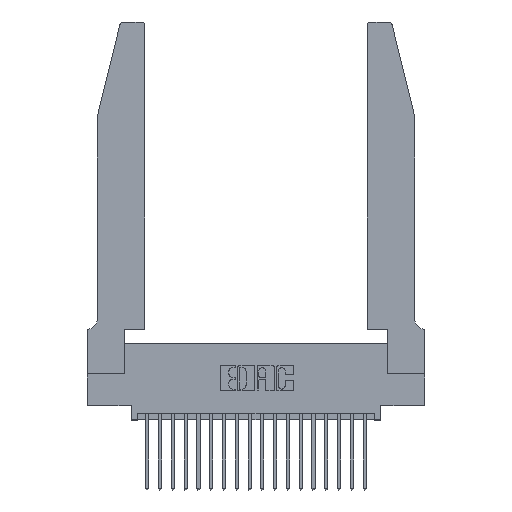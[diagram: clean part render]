
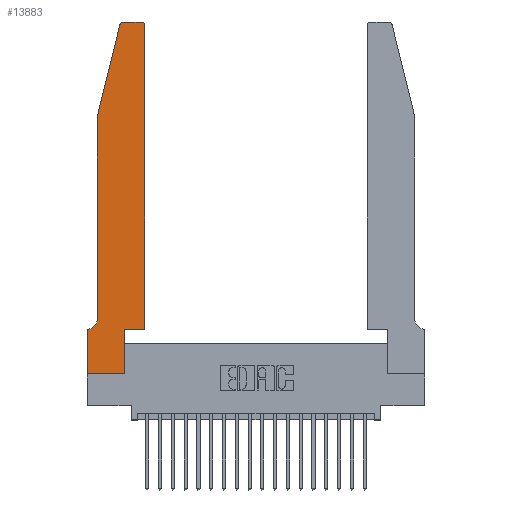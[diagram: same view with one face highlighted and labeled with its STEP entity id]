
A CAD part, top view. The second image highlights one B-rep face of the part: STEP entity #13883.
In plain terms, the highlighted planar face has unit normal (0, 0, 1).
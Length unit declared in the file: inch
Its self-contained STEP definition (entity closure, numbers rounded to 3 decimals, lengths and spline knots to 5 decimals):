
#128 = CARTESIAN_POINT ( 'NONE',  ( 0., 0.35, 0.37 ) ) ;
#136 = EDGE_CURVE ( 'NONE', #1416, #998, #16608, .T. ) ;
#261 = AXIS2_PLACEMENT_3D ( 'NONE', #13295, #6461, #11651 ) ;
#364 = VECTOR ( 'NONE', #13575, 39.37008 ) ;
#492 = VECTOR ( 'NONE', #21256, 39.37008 ) ;
#529 = DIRECTION ( 'NONE',  ( 1., 0., 0. ) ) ;
#576 = ORIENTED_EDGE ( 'NONE', *, *, #10996, .T. ) ;
#998 = VERTEX_POINT ( 'NONE', #2997 ) ;
#1009 = CARTESIAN_POINT ( 'NONE',  ( 0.284, 2.75, 0.37 ) ) ;
#1416 = VERTEX_POINT ( 'NONE', #128 ) ;
#1427 = DIRECTION ( 'NONE',  ( 0., 0., -1. ) ) ;
#1960 = CARTESIAN_POINT ( 'NONE',  ( 0.4505, 2.72, 0.37 ) ) ;
#2762 = EDGE_CURVE ( 'NONE', #20988, #3306, #14100, .T. ) ;
#2997 = CARTESIAN_POINT ( 'NONE',  ( 0., 0., 0.37 ) ) ;
#3073 = DIRECTION ( 'NONE',  ( -1., 0., 0. ) ) ;
#3126 = CARTESIAN_POINT ( 'NONE',  ( 0.0755, 0.35, 0.37 ) ) ;
#3306 = VERTEX_POINT ( 'NONE', #5013 ) ;
#3954 = CARTESIAN_POINT ( 'NONE',  ( 0.25487, 2.72718, 0.37 ) ) ;
#4302 = ORIENTED_EDGE ( 'NONE', *, *, #16537, .T. ) ;
#4662 = VERTEX_POINT ( 'NONE', #20462 ) ;
#4788 = VERTEX_POINT ( 'NONE', #1009 ) ;
#5013 = CARTESIAN_POINT ( 'NONE',  ( 0.2865, 0.35, 0.37 ) ) ;
#5222 = ORIENTED_EDGE ( 'NONE', *, *, #2762, .T. ) ;
#5242 = DIRECTION ( 'NONE',  ( -1., 0., 0. ) ) ;
#5461 = CARTESIAN_POINT ( 'NONE',  ( 0.2865, 0., 0.37 ) ) ;
#5582 = CARTESIAN_POINT ( 'NONE',  ( 0.4205, 2.75, 0.37 ) ) ;
#5585 = LINE ( 'NONE', #14156, #22278 ) ;
#5798 = ORIENTED_EDGE ( 'NONE', *, *, #12582, .T. ) ;
#5833 = CARTESIAN_POINT ( 'NONE',  ( 0.0755, 2., 0.37 ) ) ;
#6042 = DIRECTION ( 'NONE',  ( 1., 0., 0. ) ) ;
#6139 = AXIS2_PLACEMENT_3D ( 'NONE', #9614, #9840, #6042 ) ;
#6378 = EDGE_CURVE ( 'NONE', #6432, #14214, #9953, .T. ) ;
#6432 = VERTEX_POINT ( 'NONE', #11561 ) ;
#6461 = DIRECTION ( 'NONE',  ( 0., 0., 1. ) ) ;
#6501 = ORIENTED_EDGE ( 'NONE', *, *, #14180, .T. ) ;
#6626 = VECTOR ( 'NONE', #8017, 39.37008 ) ;
#7224 = CIRCLE ( 'NONE', #6139, 0.03 ) ;
#7790 = VECTOR ( 'NONE', #12864, 39.37008 ) ;
#8017 = DIRECTION ( 'NONE',  ( 0., 1., 0. ) ) ;
#8589 = FACE_OUTER_BOUND ( 'NONE', #19933, .T. ) ;
#8758 = CARTESIAN_POINT ( 'NONE',  ( 0.4505, 0.35, 0.37 ) ) ;
#9532 = VERTEX_POINT ( 'NONE', #1960 ) ;
#9598 = ORIENTED_EDGE ( 'NONE', *, *, #136, .T. ) ;
#9614 = CARTESIAN_POINT ( 'NONE',  ( 0.284, 2.72, 0.37 ) ) ;
#9824 = VERTEX_POINT ( 'NONE', #3954 ) ;
#9840 = DIRECTION ( 'NONE',  ( 0., 0., 1. ) ) ;
#9953 = CIRCLE ( 'NONE', #19726, 0.07 ) ;
#10314 = VECTOR ( 'NONE', #11611, 39.37008 ) ;
#10806 = VECTOR ( 'NONE', #14399, 39.37008 ) ;
#10824 = DIRECTION ( 'NONE',  ( -0.239, -0.971, 0. ) ) ;
#10859 = DIRECTION ( 'NONE',  ( 0., 0., 1. ) ) ;
#10996 = EDGE_CURVE ( 'NONE', #3306, #4662, #14779, .T. ) ;
#11364 = AXIS2_PLACEMENT_3D ( 'NONE', #21187, #10859, #529 ) ;
#11561 = CARTESIAN_POINT ( 'NONE',  ( 0.0755, 0.42, 0.37 ) ) ;
#11611 = DIRECTION ( 'NONE',  ( -1., 0., 0. ) ) ;
#11651 = DIRECTION ( 'NONE',  ( 1., 0., 0. ) ) ;
#12124 = ORIENTED_EDGE ( 'NONE', *, *, #14406, .T. ) ;
#12183 = LINE ( 'NONE', #20242, #364 ) ;
#12512 = DIRECTION ( 'NONE',  ( 0., -1., 0. ) ) ;
#12582 = EDGE_CURVE ( 'NONE', #4662, #9532, #18779, .T. ) ;
#12770 = VERTEX_POINT ( 'NONE', #13417 ) ;
#12864 = DIRECTION ( 'NONE',  ( 0., -1., 0. ) ) ;
#12946 = ORIENTED_EDGE ( 'NONE', *, *, #20002, .T. ) ;
#13025 = EDGE_CURVE ( 'NONE', #4788, #9824, #7224, .T. ) ;
#13295 = CARTESIAN_POINT ( 'NONE',  ( 0., 0.35, 0.37 ) ) ;
#13400 = CARTESIAN_POINT ( 'NONE',  ( 0.2865, 0.35, 0.37 ) ) ;
#13417 = CARTESIAN_POINT ( 'NONE',  ( 0.0755, 2., 0.37 ) ) ;
#13575 = DIRECTION ( 'NONE',  ( 1., 0., 0. ) ) ;
#13883 = ADVANCED_FACE ( 'NONE', ( #8589 ), #14917, .T. ) ;
#14091 = EDGE_CURVE ( 'NONE', #9532, #19957, #15506, .T. ) ;
#14100 = LINE ( 'NONE', #13400, #6626 ) ;
#14156 = CARTESIAN_POINT ( 'NONE',  ( 0.2605, 2.75, 0.37 ) ) ;
#14180 = EDGE_CURVE ( 'NONE', #19957, #4788, #5585, .T. ) ;
#14214 = VERTEX_POINT ( 'NONE', #19275 ) ;
#14216 = ORIENTED_EDGE ( 'NONE', *, *, #6378, .T. ) ;
#14304 = CARTESIAN_POINT ( 'NONE',  ( 0., 0., 0.37 ) ) ;
#14399 = DIRECTION ( 'NONE',  ( 1., 0., 0. ) ) ;
#14406 = EDGE_CURVE ( 'NONE', #9824, #12770, #15755, .T. ) ;
#14556 = CARTESIAN_POINT ( 'NONE',  ( 0.0755, 2., 0.37 ) ) ;
#14779 = LINE ( 'NONE', #19745, #10806 ) ;
#14807 = LINE ( 'NONE', #3126, #10314 ) ;
#14917 = PLANE ( 'NONE',  #261 ) ;
#15093 = ORIENTED_EDGE ( 'NONE', *, *, #13025, .T. ) ;
#15506 = CIRCLE ( 'NONE', #11364, 0.03 ) ;
#15755 = LINE ( 'NONE', #5833, #18741 ) ;
#16537 = EDGE_CURVE ( 'NONE', #998, #20988, #12183, .T. ) ;
#16608 = LINE ( 'NONE', #14304, #17135 ) ;
#17135 = VECTOR ( 'NONE', #12512, 39.37008 ) ;
#17519 = ORIENTED_EDGE ( 'NONE', *, *, #14091, .T. ) ;
#17531 = ORIENTED_EDGE ( 'NONE', *, *, #17741, .T. ) ;
#17741 = EDGE_CURVE ( 'NONE', #14214, #1416, #14807, .T. ) ;
#17944 = LINE ( 'NONE', #14556, #7790 ) ;
#18465 = CARTESIAN_POINT ( 'NONE',  ( 0.0055, 0.42, 0.37 ) ) ;
#18741 = VECTOR ( 'NONE', #10824, 39.37008 ) ;
#18779 = LINE ( 'NONE', #8758, #492 ) ;
#19275 = CARTESIAN_POINT ( 'NONE',  ( 0.0055, 0.35, 0.37 ) ) ;
#19726 = AXIS2_PLACEMENT_3D ( 'NONE', #18465, #1427, #3073 ) ;
#19745 = CARTESIAN_POINT ( 'NONE',  ( 0.4505, 0.35, 0.37 ) ) ;
#19933 = EDGE_LOOP ( 'NONE', ( #6501, #15093, #12124, #12946, #14216, #17531, #9598, #4302, #5222, #576, #5798, #17519 ) ) ;
#19957 = VERTEX_POINT ( 'NONE', #5582 ) ;
#20002 = EDGE_CURVE ( 'NONE', #12770, #6432, #17944, .T. ) ;
#20242 = CARTESIAN_POINT ( 'NONE',  ( 0., 0., 0.37 ) ) ;
#20462 = CARTESIAN_POINT ( 'NONE',  ( 0.4505, 0.35, 0.37 ) ) ;
#20988 = VERTEX_POINT ( 'NONE', #5461 ) ;
#21187 = CARTESIAN_POINT ( 'NONE',  ( 0.4205, 2.72, 0.37 ) ) ;
#21256 = DIRECTION ( 'NONE',  ( 0., 1., 0. ) ) ;
#22278 = VECTOR ( 'NONE', #5242, 39.37008 ) ;
